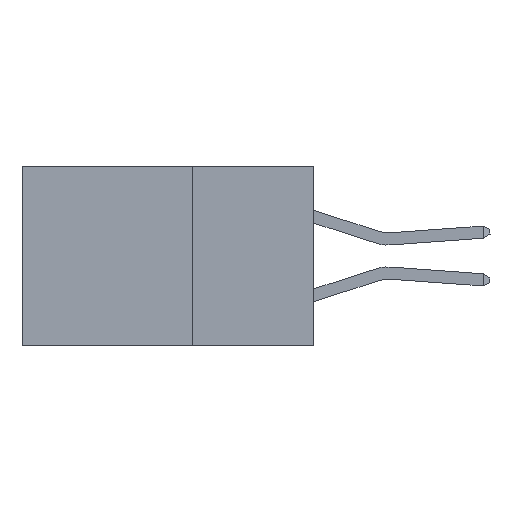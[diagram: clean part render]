
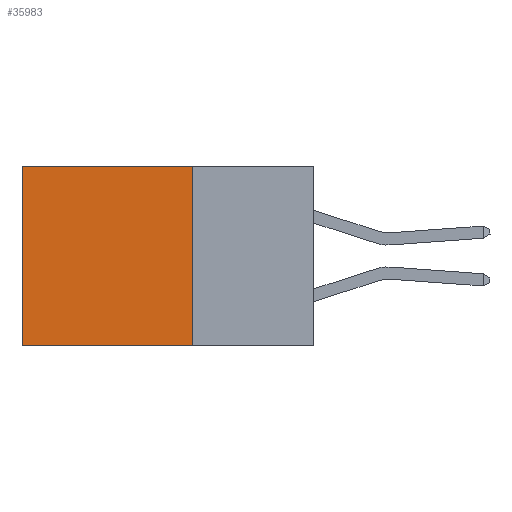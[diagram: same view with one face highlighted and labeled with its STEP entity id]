
A CAD part, left-side view. The second image highlights one B-rep face of the part: STEP entity #35983.
In plain terms, the highlighted planar face has unit normal (-1, 0, 0).
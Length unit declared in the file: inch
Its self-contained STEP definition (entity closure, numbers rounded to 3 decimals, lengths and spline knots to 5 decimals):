
#137 = AXIS2_PLACEMENT_3D ( 'NONE', #11607, #20046, #32011 ) ;
#359 = CARTESIAN_POINT ( 'NONE',  ( 0.2875, 0.25, 0. ) ) ;
#613 = CARTESIAN_POINT ( 'NONE',  ( 0.2875, 0.25, 0. ) ) ;
#1734 = EDGE_CURVE ( 'NONE', #22767, #9263, #30349, .T. ) ;
#1804 = VERTEX_POINT ( 'NONE', #34824 ) ;
#1937 = VECTOR ( 'NONE', #15439, 39.37008 ) ;
#3498 = CARTESIAN_POINT ( 'NONE',  ( 0.2875, 0.6, 0. ) ) ;
#3613 = CARTESIAN_POINT ( 'NONE',  ( 0.2875, 0.6, 0. ) ) ;
#4524 = CARTESIAN_POINT ( 'NONE',  ( 0.2875, 0.25, 0. ) ) ;
#5878 = DIRECTION ( 'NONE',  ( 0., 1., 0. ) ) ;
#9263 = VERTEX_POINT ( 'NONE', #11978 ) ;
#10119 = VECTOR ( 'NONE', #15314, 39.37008 ) ;
#10951 = EDGE_LOOP ( 'NONE', ( #35509, #33709, #38405, #28197 ) ) ;
#11420 = FACE_OUTER_BOUND ( 'NONE', #10951, .T. ) ;
#11607 = CARTESIAN_POINT ( 'NONE',  ( 0.2875, 0.25, 0. ) ) ;
#11978 = CARTESIAN_POINT ( 'NONE',  ( 0.2875, 0.6, -0.37 ) ) ;
#13148 = LINE ( 'NONE', #4524, #36769 ) ;
#15314 = DIRECTION ( 'NONE',  ( 0., 0., -1. ) ) ;
#15439 = DIRECTION ( 'NONE',  ( 0., 0., -1. ) ) ;
#15462 = EDGE_CURVE ( 'NONE', #26446, #22767, #13148, .T. ) ;
#19127 = EDGE_CURVE ( 'NONE', #1804, #9263, #35856, .T. ) ;
#20046 = DIRECTION ( 'NONE',  ( 1., 0., 0. ) ) ;
#22062 = EDGE_CURVE ( 'NONE', #26446, #1804, #30804, .T. ) ;
#22767 = VERTEX_POINT ( 'NONE', #3613 ) ;
#26446 = VERTEX_POINT ( 'NONE', #359 ) ;
#28197 = ORIENTED_EDGE ( 'NONE', *, *, #15462, .T. ) ;
#28265 = DIRECTION ( 'NONE',  ( 0., 1., 0. ) ) ;
#30349 = LINE ( 'NONE', #3498, #1937 ) ;
#30722 = VECTOR ( 'NONE', #5878, 39.37008 ) ;
#30804 = LINE ( 'NONE', #613, #10119 ) ;
#32011 = DIRECTION ( 'NONE',  ( 0., 0., -1. ) ) ;
#32336 = CARTESIAN_POINT ( 'NONE',  ( 0.2875, 0.25, -0.37 ) ) ;
#33709 = ORIENTED_EDGE ( 'NONE', *, *, #19127, .F. ) ;
#34824 = CARTESIAN_POINT ( 'NONE',  ( 0.2875, 0.25, -0.37 ) ) ;
#35509 = ORIENTED_EDGE ( 'NONE', *, *, #1734, .T. ) ;
#35856 = LINE ( 'NONE', #32336, #30722 ) ;
#35983 = ADVANCED_FACE ( 'NONE', ( #11420 ), #37876, .F. ) ;
#36769 = VECTOR ( 'NONE', #28265, 39.37008 ) ;
#37876 = PLANE ( 'NONE',  #137 ) ;
#38405 = ORIENTED_EDGE ( 'NONE', *, *, #22062, .F. ) ;
